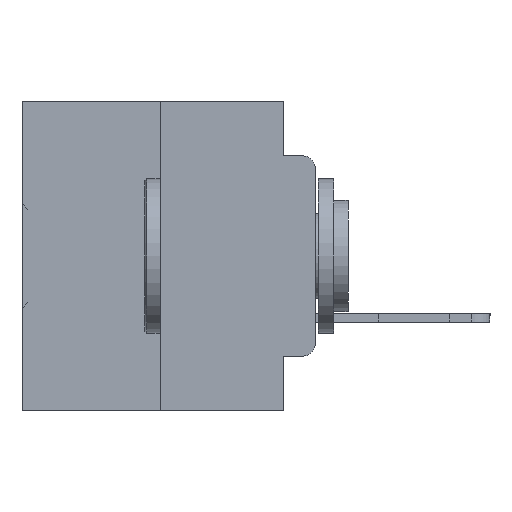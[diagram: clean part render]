
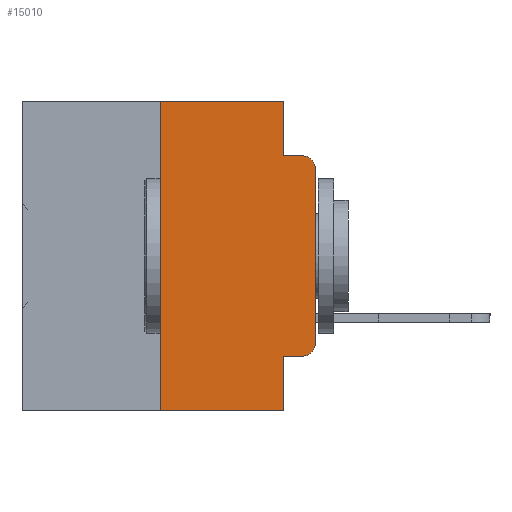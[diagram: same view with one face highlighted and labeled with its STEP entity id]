
A CAD part, left-side view. The second image highlights one B-rep face of the part: STEP entity #15010.
In plain terms, the highlighted planar face has unit normal (-1, 0, 0).
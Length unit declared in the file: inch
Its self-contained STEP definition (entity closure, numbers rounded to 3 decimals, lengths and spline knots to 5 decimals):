
#265 = CARTESIAN_POINT ( 'NONE',  ( 0., 0., -0.3915 ) ) ;
#1026 = ORIENTED_EDGE ( 'NONE', *, *, #29563, .F. ) ;
#1083 = VERTEX_POINT ( 'NONE', #30307 ) ;
#1410 = LINE ( 'NONE', #7559, #15381 ) ;
#1773 = CARTESIAN_POINT ( 'NONE',  ( 0., 0., 0. ) ) ;
#2103 = CARTESIAN_POINT ( 'NONE',  ( 0., 0.02, -0.1085 ) ) ;
#2139 = CIRCLE ( 'NONE', #32967, 0.02 ) ;
#2422 = DIRECTION ( 'NONE',  ( 0., -1., 0. ) ) ;
#2632 = DIRECTION ( 'NONE',  ( 0., 0., -1. ) ) ;
#2666 = VERTEX_POINT ( 'NONE', #14046 ) ;
#2723 = LINE ( 'NONE', #19432, #30067 ) ;
#2903 = ORIENTED_EDGE ( 'NONE', *, *, #25597, .F. ) ;
#3282 = AXIS2_PLACEMENT_3D ( 'NONE', #7398, #26444, #10164 ) ;
#4035 = LINE ( 'NONE', #1773, #18726 ) ;
#4564 = ORIENTED_EDGE ( 'NONE', *, *, #10661, .T. ) ;
#4845 = LINE ( 'NONE', #12937, #25813 ) ;
#4965 = DIRECTION ( 'NONE',  ( 0., 0., -1. ) ) ;
#5316 = VERTEX_POINT ( 'NONE', #14279 ) ;
#5494 = FACE_OUTER_BOUND ( 'NONE', #16047, .T. ) ;
#5581 = ORIENTED_EDGE ( 'NONE', *, *, #7527, .T. ) ;
#5902 = ORIENTED_EDGE ( 'NONE', *, *, #12736, .F. ) ;
#7374 = VERTEX_POINT ( 'NONE', #265 ) ;
#7398 = CARTESIAN_POINT ( 'NONE',  ( 0., 0.02, -0.3915 ) ) ;
#7527 = EDGE_CURVE ( 'NONE', #9591, #19796, #33144, .T. ) ;
#7559 = CARTESIAN_POINT ( 'NONE',  ( 0., 0.051, 0. ) ) ;
#7690 = DIRECTION ( 'NONE',  ( 0., -1., 0. ) ) ;
#8373 = DIRECTION ( 'NONE',  ( 0., 0., 1. ) ) ;
#9271 = CARTESIAN_POINT ( 'NONE',  ( 0., 0.051, -0.4115 ) ) ;
#9483 = CARTESIAN_POINT ( 'NONE',  ( 0., 0.25, -0.5 ) ) ;
#9591 = VERTEX_POINT ( 'NONE', #23658 ) ;
#10164 = DIRECTION ( 'NONE',  ( 0., 0., -1. ) ) ;
#10168 = DIRECTION ( 'NONE',  ( 0., -1., 0. ) ) ;
#10234 = PLANE ( 'NONE',  #30192 ) ;
#10661 = EDGE_CURVE ( 'NONE', #7374, #2666, #4035, .T. ) ;
#11507 = CARTESIAN_POINT ( 'NONE',  ( 0., 0.02, -0.0885 ) ) ;
#11643 = ORIENTED_EDGE ( 'NONE', *, *, #16542, .T. ) ;
#12736 = EDGE_CURVE ( 'NONE', #5316, #23635, #26980, .T. ) ;
#12937 = CARTESIAN_POINT ( 'NONE',  ( 0., 0.473, -0.5 ) ) ;
#13011 = DIRECTION ( 'NONE',  ( 1., 0., 0. ) ) ;
#13666 = ORIENTED_EDGE ( 'NONE', *, *, #19295, .T. ) ;
#14046 = CARTESIAN_POINT ( 'NONE',  ( 0., 0., -0.1085 ) ) ;
#14279 = CARTESIAN_POINT ( 'NONE',  ( 0., 0.051, -0.0885 ) ) ;
#15010 = ADVANCED_FACE ( 'NONE', ( #5494 ), #10234, .F. ) ;
#15381 = VECTOR ( 'NONE', #15891, 39.37008 ) ;
#15891 = DIRECTION ( 'NONE',  ( 0., 0., -1. ) ) ;
#16047 = EDGE_LOOP ( 'NONE', ( #4564, #13666, #5902, #1026, #20162, #34740, #29364, #2903, #5581, #11643 ) ) ;
#16449 = VERTEX_POINT ( 'NONE', #9483 ) ;
#16542 = EDGE_CURVE ( 'NONE', #19796, #7374, #20153, .T. ) ;
#17597 = DIRECTION ( 'NONE',  ( 0., -1., 0. ) ) ;
#17818 = VERTEX_POINT ( 'NONE', #30189 ) ;
#18473 = CARTESIAN_POINT ( 'NONE',  ( 0., 0.02, -0.4115 ) ) ;
#18726 = VECTOR ( 'NONE', #21154, 39.37008 ) ;
#18936 = VECTOR ( 'NONE', #17597, 39.37008 ) ;
#19037 = CARTESIAN_POINT ( 'NONE',  ( 0., 0.473, 0. ) ) ;
#19293 = VERTEX_POINT ( 'NONE', #29371 ) ;
#19295 = EDGE_CURVE ( 'NONE', #2666, #23635, #2139, .T. ) ;
#19432 = CARTESIAN_POINT ( 'NONE',  ( 0., 0.25, 0. ) ) ;
#19796 = VERTEX_POINT ( 'NONE', #18473 ) ;
#19859 = VECTOR ( 'NONE', #7690, 39.37008 ) ;
#20153 = CIRCLE ( 'NONE', #3282, 0.02 ) ;
#20162 = ORIENTED_EDGE ( 'NONE', *, *, #32018, .F. ) ;
#21154 = DIRECTION ( 'NONE',  ( 0., 0., 1. ) ) ;
#21454 = DIRECTION ( 'NONE',  ( -1., 0., 0. ) ) ;
#21544 = LINE ( 'NONE', #35166, #28645 ) ;
#23635 = VERTEX_POINT ( 'NONE', #11507 ) ;
#23658 = CARTESIAN_POINT ( 'NONE',  ( 0., 0.051, -0.4115 ) ) ;
#24026 = CARTESIAN_POINT ( 'NONE',  ( 0., 0.051, -0.0885 ) ) ;
#25597 = EDGE_CURVE ( 'NONE', #9591, #17818, #1410, .T. ) ;
#25788 = EDGE_CURVE ( 'NONE', #16449, #19293, #2723, .T. ) ;
#25813 = VECTOR ( 'NONE', #10168, 39.37008 ) ;
#26444 = DIRECTION ( 'NONE',  ( -1., 0., 0. ) ) ;
#26980 = LINE ( 'NONE', #24026, #19859 ) ;
#27359 = VECTOR ( 'NONE', #2422, 39.37008 ) ;
#28052 = EDGE_CURVE ( 'NONE', #16449, #17818, #4845, .T. ) ;
#28645 = VECTOR ( 'NONE', #2632, 39.37008 ) ;
#29364 = ORIENTED_EDGE ( 'NONE', *, *, #28052, .T. ) ;
#29371 = CARTESIAN_POINT ( 'NONE',  ( 0., 0.25, 0. ) ) ;
#29563 = EDGE_CURVE ( 'NONE', #1083, #5316, #21544, .T. ) ;
#30067 = VECTOR ( 'NONE', #8373, 39.37008 ) ;
#30189 = CARTESIAN_POINT ( 'NONE',  ( 0., 0.051, -0.5 ) ) ;
#30192 = AXIS2_PLACEMENT_3D ( 'NONE', #34407, #13011, #31836 ) ;
#30307 = CARTESIAN_POINT ( 'NONE',  ( 0., 0.051, 0. ) ) ;
#31836 = DIRECTION ( 'NONE',  ( 0., 0., -1. ) ) ;
#32018 = EDGE_CURVE ( 'NONE', #19293, #1083, #34036, .T. ) ;
#32967 = AXIS2_PLACEMENT_3D ( 'NONE', #2103, #21454, #4965 ) ;
#33144 = LINE ( 'NONE', #9271, #18936 ) ;
#34036 = LINE ( 'NONE', #19037, #27359 ) ;
#34407 = CARTESIAN_POINT ( 'NONE',  ( 0., 0.473, 0. ) ) ;
#34740 = ORIENTED_EDGE ( 'NONE', *, *, #25788, .F. ) ;
#35166 = CARTESIAN_POINT ( 'NONE',  ( 0., 0.051, 0. ) ) ;
